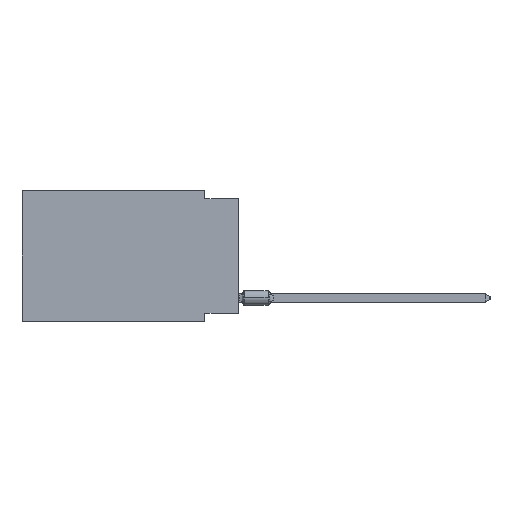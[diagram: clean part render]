
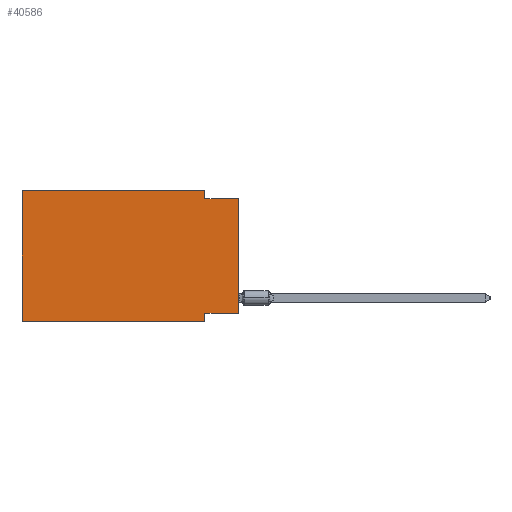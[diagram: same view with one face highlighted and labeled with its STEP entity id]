
A CAD part, left-side view. The second image highlights one B-rep face of the part: STEP entity #40586.
In plain terms, the highlighted planar face has unit normal (-1, 0, 0).
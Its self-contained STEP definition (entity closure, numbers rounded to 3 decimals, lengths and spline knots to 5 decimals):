
#1292 = VERTEX_POINT ( 'NONE', #2729 ) ;
#1624 = LINE ( 'NONE', #15448, #87998 ) ;
#2220 = CARTESIAN_POINT ( 'NONE',  ( 0., 0., -0.365 ) ) ;
#2412 = CARTESIAN_POINT ( 'NONE',  ( 0., 0.645, 0. ) ) ;
#2483 = EDGE_LOOP ( 'NONE', ( #9615, #79196, #8295, #29331, #52417, #16234, #78145, #13131 ) ) ;
#2729 = CARTESIAN_POINT ( 'NONE',  ( 0., 0.645, -0.39 ) ) ;
#4683 = FACE_OUTER_BOUND ( 'NONE', #2483, .T. ) ;
#8295 = ORIENTED_EDGE ( 'NONE', *, *, #21573, .F. ) ;
#9615 = ORIENTED_EDGE ( 'NONE', *, *, #50909, .T. ) ;
#10174 = DIRECTION ( 'NONE',  ( 0., -1., 0. ) ) ;
#11877 = CARTESIAN_POINT ( 'NONE',  ( 0., 0.1, 0. ) ) ;
#11998 = EDGE_CURVE ( 'NONE', #39319, #78114, #46603, .T. ) ;
#12108 = DIRECTION ( 'NONE',  ( 0., 0., 1. ) ) ;
#12750 = DIRECTION ( 'NONE',  ( 0., 0., -1. ) ) ;
#13131 = ORIENTED_EDGE ( 'NONE', *, *, #64194, .F. ) ;
#15092 = VECTOR ( 'NONE', #68792, 39.37008 ) ;
#15448 = CARTESIAN_POINT ( 'NONE',  ( 0., 0., 0. ) ) ;
#16234 = ORIENTED_EDGE ( 'NONE', *, *, #87025, .T. ) ;
#17296 = CARTESIAN_POINT ( 'NONE',  ( 0., 0.645, -0.39 ) ) ;
#18815 = EDGE_CURVE ( 'NONE', #1292, #87576, #78076, .T. ) ;
#18935 = CARTESIAN_POINT ( 'NONE',  ( 0., 0.645, 0. ) ) ;
#20770 = VECTOR ( 'NONE', #10174, 39.37008 ) ;
#21573 = EDGE_CURVE ( 'NONE', #52204, #50449, #68352, .T. ) ;
#25671 = CARTESIAN_POINT ( 'NONE',  ( 0., 0., -0.365 ) ) ;
#28666 = CARTESIAN_POINT ( 'NONE',  ( 0., 0.1, 0. ) ) ;
#29331 = ORIENTED_EDGE ( 'NONE', *, *, #41750, .F. ) ;
#30433 = VECTOR ( 'NONE', #12108, 39.37008 ) ;
#31076 = LINE ( 'NONE', #17296, #20770 ) ;
#31856 = DIRECTION ( 'NONE',  ( 1., 0., 0. ) ) ;
#32765 = VECTOR ( 'NONE', #62553, 39.37008 ) ;
#34227 = DIRECTION ( 'NONE',  ( 0., -1., 0. ) ) ;
#34676 = LINE ( 'NONE', #68091, #81997 ) ;
#35410 = EDGE_CURVE ( 'NONE', #50449, #87794, #34676, .T. ) ;
#36090 = DIRECTION ( 'NONE',  ( 0., 1., 0. ) ) ;
#36992 = VECTOR ( 'NONE', #12750, 39.37008 ) ;
#38519 = CARTESIAN_POINT ( 'NONE',  ( 0., 0.645, 0. ) ) ;
#39319 = VERTEX_POINT ( 'NONE', #56385 ) ;
#40586 = ADVANCED_FACE ( 'NONE', ( #4683 ), #46518, .F. ) ;
#41750 = EDGE_CURVE ( 'NONE', #87576, #52204, #42503, .T. ) ;
#42503 = LINE ( 'NONE', #2412, #32765 ) ;
#46518 = PLANE ( 'NONE',  #69666 ) ;
#46603 = LINE ( 'NONE', #73789, #36992 ) ;
#50449 = VERTEX_POINT ( 'NONE', #72325 ) ;
#50909 = EDGE_CURVE ( 'NONE', #80615, #87794, #1624, .T. ) ;
#52188 = CARTESIAN_POINT ( 'NONE',  ( 0., 0.645, 0. ) ) ;
#52204 = VERTEX_POINT ( 'NONE', #11877 ) ;
#52417 = ORIENTED_EDGE ( 'NONE', *, *, #18815, .F. ) ;
#53051 = VECTOR ( 'NONE', #36090, 39.37008 ) ;
#56385 = CARTESIAN_POINT ( 'NONE',  ( 0., 0.1, -0.365 ) ) ;
#57031 = LINE ( 'NONE', #2220, #53051 ) ;
#59026 = DIRECTION ( 'NONE',  ( 0., 0., -1. ) ) ;
#62553 = DIRECTION ( 'NONE',  ( 0., -1., 0. ) ) ;
#63122 = DIRECTION ( 'NONE',  ( 0., 0., 1. ) ) ;
#64194 = EDGE_CURVE ( 'NONE', #80615, #39319, #57031, .T. ) ;
#68091 = CARTESIAN_POINT ( 'NONE',  ( 0., 0., -0.025 ) ) ;
#68352 = LINE ( 'NONE', #28666, #15092 ) ;
#68792 = DIRECTION ( 'NONE',  ( 0., 0., -1. ) ) ;
#69666 = AXIS2_PLACEMENT_3D ( 'NONE', #38519, #31856, #59026 ) ;
#70555 = CARTESIAN_POINT ( 'NONE',  ( 0., 0., -0.025 ) ) ;
#72298 = CARTESIAN_POINT ( 'NONE',  ( 0., 0.1, -0.39 ) ) ;
#72325 = CARTESIAN_POINT ( 'NONE',  ( 0., 0.1, -0.025 ) ) ;
#73789 = CARTESIAN_POINT ( 'NONE',  ( 0., 0.1, -0.39 ) ) ;
#78076 = LINE ( 'NONE', #52188, #30433 ) ;
#78114 = VERTEX_POINT ( 'NONE', #72298 ) ;
#78145 = ORIENTED_EDGE ( 'NONE', *, *, #11998, .F. ) ;
#79196 = ORIENTED_EDGE ( 'NONE', *, *, #35410, .F. ) ;
#80615 = VERTEX_POINT ( 'NONE', #25671 ) ;
#81997 = VECTOR ( 'NONE', #34227, 39.37008 ) ;
#87025 = EDGE_CURVE ( 'NONE', #1292, #78114, #31076, .T. ) ;
#87576 = VERTEX_POINT ( 'NONE', #18935 ) ;
#87794 = VERTEX_POINT ( 'NONE', #70555 ) ;
#87998 = VECTOR ( 'NONE', #63122, 39.37008 ) ;
